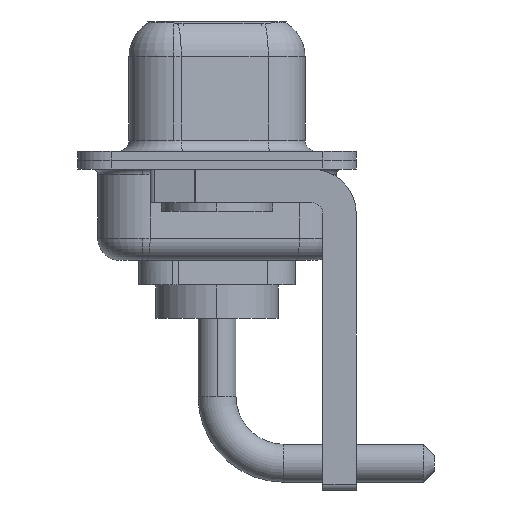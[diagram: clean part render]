
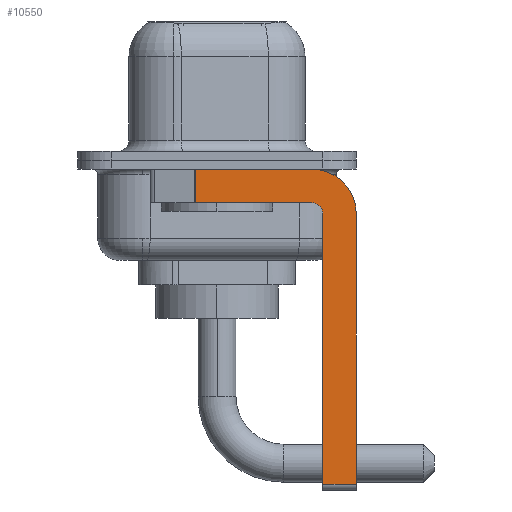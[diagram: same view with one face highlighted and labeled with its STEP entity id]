
A CAD part, left-side view. The second image highlights one B-rep face of the part: STEP entity #10550.
In plain terms, the highlighted planar face has unit normal (-1, 0, 0).
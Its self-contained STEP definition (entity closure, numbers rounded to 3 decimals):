
#175 = VECTOR ( 'NONE', #8949, 1000. ) ;
#539 = DIRECTION ( 'NONE',  ( -1., 0., 0. ) ) ;
#593 = VECTOR ( 'NONE', #7798, 1000. ) ;
#601 = DIRECTION ( 'NONE',  ( 0., 0., 1. ) ) ;
#765 = PLANE ( 'NONE',  #9380 ) ;
#779 = ORIENTED_EDGE ( 'NONE', *, *, #8470, .F. ) ;
#890 = DIRECTION ( 'NONE',  ( 1., 0., 0. ) ) ;
#1053 = VERTEX_POINT ( 'NONE', #8059 ) ;
#1080 = EDGE_CURVE ( 'NONE', #8935, #1053, #1317, .T. ) ;
#1142 = DIRECTION ( 'NONE',  ( 0., 1., 0. ) ) ;
#1317 = CIRCLE ( 'NONE', #12351, 0.5 ) ;
#1509 = CARTESIAN_POINT ( 'NONE',  ( -2.9, -6.25, -14.55 ) ) ;
#1545 = ORIENTED_EDGE ( 'NONE', *, *, #5808, .F. ) ;
#2158 = CARTESIAN_POINT ( 'NONE',  ( -2.9, -6.25, -2.4 ) ) ;
#2474 = CARTESIAN_POINT ( 'NONE',  ( -2.9, 0.978, -1.9 ) ) ;
#2481 = VERTEX_POINT ( 'NONE', #1509 ) ;
#2505 = LINE ( 'NONE', #9298, #5355 ) ;
#2613 = VERTEX_POINT ( 'NONE', #2686 ) ;
#2686 = CARTESIAN_POINT ( 'NONE',  ( -2.9, 0.978, -0.4 ) ) ;
#2872 = VERTEX_POINT ( 'NONE', #10430 ) ;
#3106 = CARTESIAN_POINT ( 'NONE',  ( -2.9, -4.75, -2.4 ) ) ;
#3120 = LINE ( 'NONE', #5168, #12402 ) ;
#3192 = CARTESIAN_POINT ( 'NONE',  ( -2.9, -4.25, -14.55 ) ) ;
#3312 = ORIENTED_EDGE ( 'NONE', *, *, #5270, .F. ) ;
#3393 = ORIENTED_EDGE ( 'NONE', *, *, #12764, .F. ) ;
#3588 = EDGE_LOOP ( 'NONE', ( #3312, #4514, #1545, #6637, #779, #4175, #9322, #3393 ) ) ;
#4175 = ORIENTED_EDGE ( 'NONE', *, *, #9865, .T. ) ;
#4232 = DIRECTION ( 'NONE',  ( 0., 0., -1. ) ) ;
#4244 = LINE ( 'NONE', #9968, #5444 ) ;
#4410 = CARTESIAN_POINT ( 'NONE',  ( -2.9, -4.25, -2.4 ) ) ;
#4514 = ORIENTED_EDGE ( 'NONE', *, *, #6465, .T. ) ;
#4534 = DIRECTION ( 'NONE',  ( 0., 0., -1. ) ) ;
#4883 = DIRECTION ( 'NONE',  ( 0., 0., -1. ) ) ;
#5168 = CARTESIAN_POINT ( 'NONE',  ( -2.9, -4.75, -14.8 ) ) ;
#5270 = EDGE_CURVE ( 'NONE', #2613, #2872, #9883, .T. ) ;
#5355 = VECTOR ( 'NONE', #8393, 1000. ) ;
#5394 = DIRECTION ( 'NONE',  ( 1., 0., 0. ) ) ;
#5444 = VECTOR ( 'NONE', #1142, 1000. ) ;
#5471 = AXIS2_PLACEMENT_3D ( 'NONE', #4410, #5394, #4534 ) ;
#5521 = CARTESIAN_POINT ( 'NONE',  ( -2.9, -4.25, -2.4 ) ) ;
#5808 = EDGE_CURVE ( 'NONE', #1053, #7306, #4244, .T. ) ;
#5873 = CARTESIAN_POINT ( 'NONE',  ( -2.9, -4.25, -2.4 ) ) ;
#5903 = EDGE_CURVE ( 'NONE', #7114, #2481, #10105, .T. ) ;
#5987 = CARTESIAN_POINT ( 'NONE',  ( -2.9, -4.75, -14.55 ) ) ;
#6034 = CARTESIAN_POINT ( 'NONE',  ( -2.9, 3., -0.4 ) ) ;
#6067 = CARTESIAN_POINT ( 'NONE',  ( -2.9, -6.25, -2.4 ) ) ;
#6200 = VERTEX_POINT ( 'NONE', #5987 ) ;
#6465 = EDGE_CURVE ( 'NONE', #2613, #7306, #2505, .T. ) ;
#6637 = ORIENTED_EDGE ( 'NONE', *, *, #1080, .F. ) ;
#7114 = VERTEX_POINT ( 'NONE', #2158 ) ;
#7306 = VERTEX_POINT ( 'NONE', #2474 ) ;
#7798 = DIRECTION ( 'NONE',  ( 0., -1., 0. ) ) ;
#8035 = DIRECTION ( 'NONE',  ( 0., 0., 1. ) ) ;
#8059 = CARTESIAN_POINT ( 'NONE',  ( -2.9, -4.25, -1.9 ) ) ;
#8393 = DIRECTION ( 'NONE',  ( 0., 0., -1. ) ) ;
#8470 = EDGE_CURVE ( 'NONE', #6200, #8935, #3120, .T. ) ;
#8935 = VERTEX_POINT ( 'NONE', #3106 ) ;
#8949 = DIRECTION ( 'NONE',  ( 0., -1., 0. ) ) ;
#9298 = CARTESIAN_POINT ( 'NONE',  ( -2.9, 0.978, -1.9 ) ) ;
#9322 = ORIENTED_EDGE ( 'NONE', *, *, #5903, .F. ) ;
#9380 = AXIS2_PLACEMENT_3D ( 'NONE', #5873, #890, #4883 ) ;
#9865 = EDGE_CURVE ( 'NONE', #6200, #2481, #10124, .T. ) ;
#9883 = LINE ( 'NONE', #6034, #593 ) ;
#9968 = CARTESIAN_POINT ( 'NONE',  ( -2.9, -4.25, -1.9 ) ) ;
#10105 = LINE ( 'NONE', #6067, #12098 ) ;
#10124 = LINE ( 'NONE', #3192, #175 ) ;
#10430 = CARTESIAN_POINT ( 'NONE',  ( -2.9, -4.25, -0.4 ) ) ;
#10550 = ADVANCED_FACE ( 'NONE', ( #12654 ), #765, .F. ) ;
#11084 = CIRCLE ( 'NONE', #5471, 2. ) ;
#12098 = VECTOR ( 'NONE', #4232, 1000. ) ;
#12351 = AXIS2_PLACEMENT_3D ( 'NONE', #5521, #539, #601 ) ;
#12402 = VECTOR ( 'NONE', #8035, 1000. ) ;
#12654 = FACE_OUTER_BOUND ( 'NONE', #3588, .T. ) ;
#12764 = EDGE_CURVE ( 'NONE', #2872, #7114, #11084, .T. ) ;
